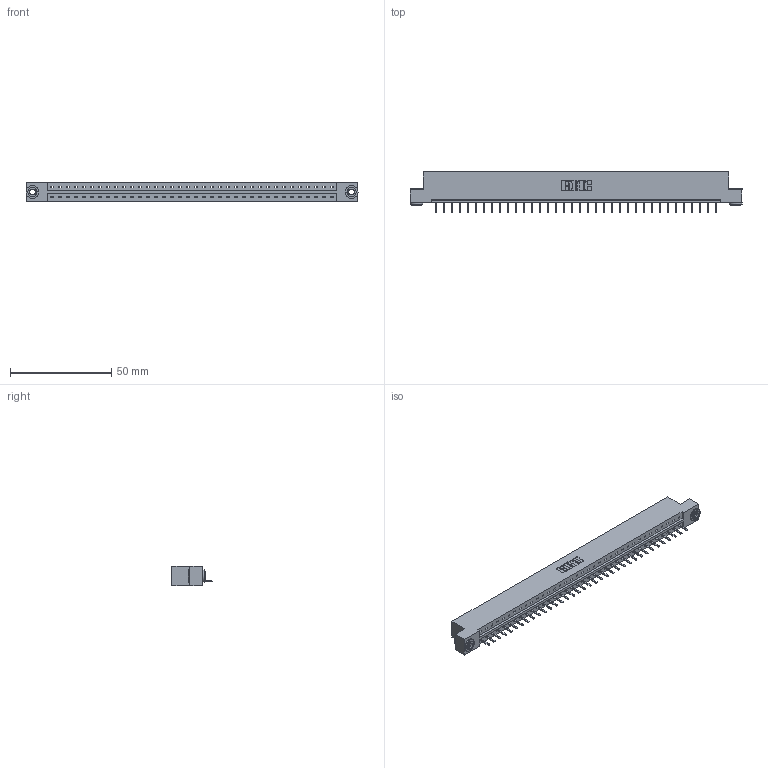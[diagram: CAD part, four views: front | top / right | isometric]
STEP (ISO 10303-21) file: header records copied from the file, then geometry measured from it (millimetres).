
FILE_DESCRIPTION (( 'STEP AP203' ), '1' );
FILE_NAME ('833-036-520-103.STEP', '2020-06-03T01:35:57', ( '' ), ( '' ), 'SwSTEP 2.0', 'SolidWorks 2020', '' );
FILE_SCHEMA (( 'CONFIG_CONTROL_DESIGN' ));
Length unit declared in the file: inch
Products named in the file (4): 345-292-001_345-293-120; 833-036-520-103; 833 Part_Flush - .156 Dia - TH; 345-250-002_345-250-002-102
Assembly tree (39 placements, depth 2):
  833-036-520-103
    833 Part_Flush - .156 Dia - TH
    345-292-001_345-293-120  x36
    345-250-002_345-250-002-102  x2
Bounding box: 164.19 x 20.02 x 9.4 mm (x, y, z)
Volume: 16385.9 mm3; surface area: 17554.4 mm2
Topology: 39 solids, 39 shells, 2384 faces, 7011 edges, 4574 vertices
Faces by surface type: plane 1664, cylinder 712, cone 8
Entity records: 23548 total; most frequent: CARTESIAN_POINT 4053, ORIENTED_EDGE 4006, DIRECTION 3453, EDGE_CURVE 2003, LINE 1847, VECTOR 1847, VERTEX_POINT 1330, AXIS2_PLACEMENT_3D 803
